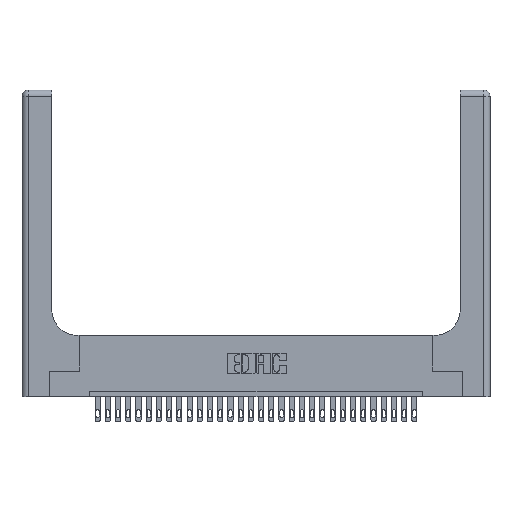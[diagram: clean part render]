
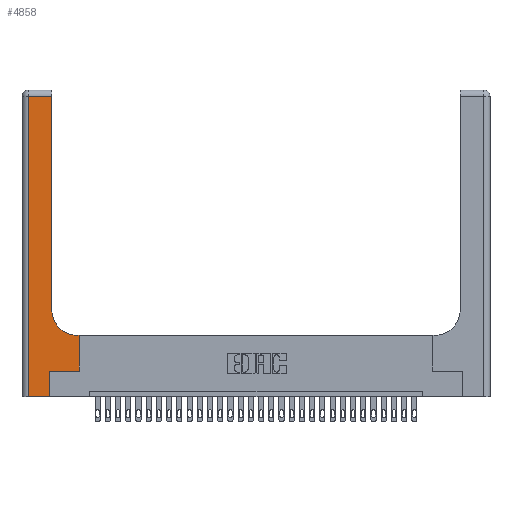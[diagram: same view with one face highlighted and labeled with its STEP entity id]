
A CAD part, top view. The second image highlights one B-rep face of the part: STEP entity #4858.
In plain terms, the highlighted planar face has unit normal (0, 0, 1).
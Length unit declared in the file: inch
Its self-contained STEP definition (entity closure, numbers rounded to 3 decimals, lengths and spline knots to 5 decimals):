
#300 = CARTESIAN_POINT ( 'NONE',  ( 0.5415, 0.6, 0.37 ) ) ;
#510 = LINE ( 'NONE', #14064, #1935 ) ;
#1101 = CARTESIAN_POINT ( 'NONE',  ( 0.2915, 3., 0.37 ) ) ;
#1671 = EDGE_CURVE ( 'NONE', #3846, #2949, #14213, .T. ) ;
#1935 = VECTOR ( 'NONE', #19139, 39.37008 ) ;
#1966 = CARTESIAN_POINT ( 'NONE',  ( 0.2915, 0.85, 0.37 ) ) ;
#2510 = EDGE_CURVE ( 'NONE', #4139, #22481, #28598, .T. ) ;
#2832 = CARTESIAN_POINT ( 'NONE',  ( 0.2915, 2.94, 0.37 ) ) ;
#2949 = VERTEX_POINT ( 'NONE', #1966 ) ;
#2975 = DIRECTION ( 'NONE',  ( 0., 1., 0. ) ) ;
#3272 = CARTESIAN_POINT ( 'NONE',  ( 0.2915, 0.6, 0.37 ) ) ;
#3846 = VERTEX_POINT ( 'NONE', #300 ) ;
#4067 = CARTESIAN_POINT ( 'NONE',  ( 0.269, 0., 0.37 ) ) ;
#4139 = VERTEX_POINT ( 'NONE', #4067 ) ;
#4269 = VECTOR ( 'NONE', #17999, 39.37008 ) ;
#4493 = CARTESIAN_POINT ( 'NONE',  ( 0.269, 0.25, 0.37 ) ) ;
#4776 = CARTESIAN_POINT ( 'NONE',  ( 0.269, 0.25, 0.37 ) ) ;
#4858 = ADVANCED_FACE ( 'NONE', ( #30286 ), #10505, .F. ) ;
#5318 = DIRECTION ( 'NONE',  ( 0., 1., 0. ) ) ;
#5528 = AXIS2_PLACEMENT_3D ( 'NONE', #17200, #7864, #24319 ) ;
#5855 = EDGE_CURVE ( 'NONE', #10567, #16217, #15478, .T. ) ;
#6194 = VERTEX_POINT ( 'NONE', #22572 ) ;
#7508 = CARTESIAN_POINT ( 'NONE',  ( 0.06, 2.94, 0.37 ) ) ;
#7601 = CARTESIAN_POINT ( 'NONE',  ( 0.269, 0., 0.37 ) ) ;
#7864 = DIRECTION ( 'NONE',  ( 0., 0., -1. ) ) ;
#7904 = ORIENTED_EDGE ( 'NONE', *, *, #1671, .T. ) ;
#7908 = ORIENTED_EDGE ( 'NONE', *, *, #22102, .T. ) ;
#9014 = ORIENTED_EDGE ( 'NONE', *, *, #25249, .T. ) ;
#10057 = LINE ( 'NONE', #4493, #15554 ) ;
#10505 = PLANE ( 'NONE',  #15416 ) ;
#10532 = LINE ( 'NONE', #27595, #4269 ) ;
#10567 = VERTEX_POINT ( 'NONE', #23911 ) ;
#11246 = VECTOR ( 'NONE', #14655, 39.37008 ) ;
#12264 = EDGE_CURVE ( 'NONE', #22481, #10567, #10057, .T. ) ;
#12341 = DIRECTION ( 'NONE',  ( -1., 0., 0. ) ) ;
#12567 = EDGE_LOOP ( 'NONE', ( #7908, #22813, #30402, #9014, #12657, #14533, #29509, #15758, #7904 ) ) ;
#12657 = ORIENTED_EDGE ( 'NONE', *, *, #2510, .T. ) ;
#12978 = VERTEX_POINT ( 'NONE', #2832 ) ;
#13836 = DIRECTION ( 'NONE',  ( 1., 0., 0. ) ) ;
#14013 = LINE ( 'NONE', #1101, #14777 ) ;
#14064 = CARTESIAN_POINT ( 'NONE',  ( 0., 2.94, 0.37 ) ) ;
#14198 = VERTEX_POINT ( 'NONE', #7508 ) ;
#14213 = CIRCLE ( 'NONE', #5528, 0.25 ) ;
#14533 = ORIENTED_EDGE ( 'NONE', *, *, #12264, .T. ) ;
#14636 = LINE ( 'NONE', #26613, #26479 ) ;
#14655 = DIRECTION ( 'NONE',  ( 0., 1., 0. ) ) ;
#14777 = VECTOR ( 'NONE', #2975, 39.37008 ) ;
#14878 = DIRECTION ( 'NONE',  ( -1., 0., 0. ) ) ;
#14915 = EDGE_CURVE ( 'NONE', #14198, #6194, #14636, .T. ) ;
#15416 = AXIS2_PLACEMENT_3D ( 'NONE', #17091, #22341, #12341 ) ;
#15478 = LINE ( 'NONE', #26331, #16216 ) ;
#15554 = VECTOR ( 'NONE', #13836, 39.37008 ) ;
#15758 = ORIENTED_EDGE ( 'NONE', *, *, #22135, .T. ) ;
#16216 = VECTOR ( 'NONE', #5318, 39.37008 ) ;
#16217 = VERTEX_POINT ( 'NONE', #29987 ) ;
#17091 = CARTESIAN_POINT ( 'NONE',  ( 0., 3., 0.37 ) ) ;
#17200 = CARTESIAN_POINT ( 'NONE',  ( 0.5415, 0.85, 0.37 ) ) ;
#17999 = DIRECTION ( 'NONE',  ( 1., 0., 0. ) ) ;
#19139 = DIRECTION ( 'NONE',  ( -1., 0., 0. ) ) ;
#22102 = EDGE_CURVE ( 'NONE', #2949, #12978, #14013, .T. ) ;
#22134 = VECTOR ( 'NONE', #14878, 39.37008 ) ;
#22135 = EDGE_CURVE ( 'NONE', #16217, #3846, #29889, .T. ) ;
#22341 = DIRECTION ( 'NONE',  ( 0., 0., -1. ) ) ;
#22481 = VERTEX_POINT ( 'NONE', #4776 ) ;
#22572 = CARTESIAN_POINT ( 'NONE',  ( 0.06, 0., 0.37 ) ) ;
#22813 = ORIENTED_EDGE ( 'NONE', *, *, #27396, .T. ) ;
#23911 = CARTESIAN_POINT ( 'NONE',  ( 0.5585, 0.25, 0.37 ) ) ;
#24319 = DIRECTION ( 'NONE',  ( 1., 0., 0. ) ) ;
#24441 = DIRECTION ( 'NONE',  ( 0., -1., 0. ) ) ;
#25249 = EDGE_CURVE ( 'NONE', #6194, #4139, #10532, .T. ) ;
#26331 = CARTESIAN_POINT ( 'NONE',  ( 0.5585, 0.25, 0.37 ) ) ;
#26479 = VECTOR ( 'NONE', #24441, 39.37008 ) ;
#26613 = CARTESIAN_POINT ( 'NONE',  ( 0.06, 3., 0.37 ) ) ;
#27396 = EDGE_CURVE ( 'NONE', #12978, #14198, #510, .T. ) ;
#27595 = CARTESIAN_POINT ( 'NONE',  ( 0., 0., 0.37 ) ) ;
#28598 = LINE ( 'NONE', #7601, #11246 ) ;
#29509 = ORIENTED_EDGE ( 'NONE', *, *, #5855, .T. ) ;
#29889 = LINE ( 'NONE', #3272, #22134 ) ;
#29987 = CARTESIAN_POINT ( 'NONE',  ( 0.5585, 0.6, 0.37 ) ) ;
#30286 = FACE_OUTER_BOUND ( 'NONE', #12567, .T. ) ;
#30402 = ORIENTED_EDGE ( 'NONE', *, *, #14915, .T. ) ;
